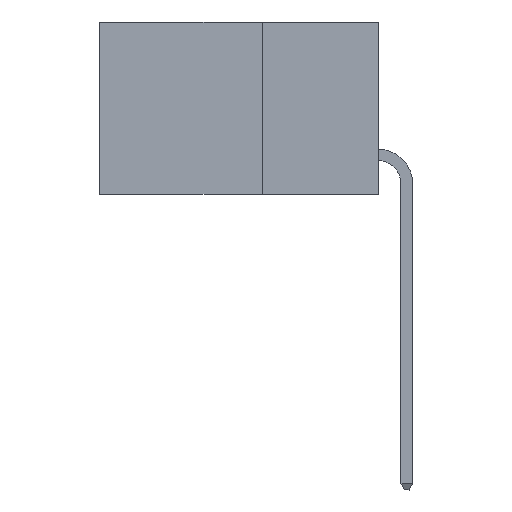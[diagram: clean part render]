
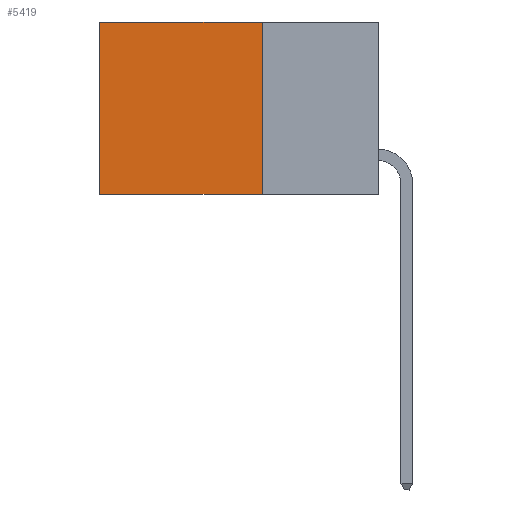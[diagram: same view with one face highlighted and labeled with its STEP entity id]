
A CAD part, left-side view. The second image highlights one B-rep face of the part: STEP entity #5419.
In plain terms, the highlighted planar face has unit normal (-1, 0, 0).
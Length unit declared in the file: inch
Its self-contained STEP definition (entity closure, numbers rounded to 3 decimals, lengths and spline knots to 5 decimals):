
#179 = VERTEX_POINT ( 'NONE', #9952 ) ;
#425 = DIRECTION ( 'NONE',  ( 0., 0., -1. ) ) ;
#601 = CARTESIAN_POINT ( 'NONE',  ( 0.298, 0.25, 0. ) ) ;
#1178 = VERTEX_POINT ( 'NONE', #8775 ) ;
#1567 = ORIENTED_EDGE ( 'NONE', *, *, #10759, .F. ) ;
#2177 = CARTESIAN_POINT ( 'NONE',  ( 0.298, 0.25, -0.37 ) ) ;
#2369 = VECTOR ( 'NONE', #10556, 39.37008 ) ;
#2895 = VERTEX_POINT ( 'NONE', #9377 ) ;
#3828 = CARTESIAN_POINT ( 'NONE',  ( 0.298, 0.25, 0. ) ) ;
#3867 = CARTESIAN_POINT ( 'NONE',  ( 0.298, 0.25, 0. ) ) ;
#4119 = FACE_OUTER_BOUND ( 'NONE', #5281, .T. ) ;
#4144 = LINE ( 'NONE', #7841, #4399 ) ;
#4399 = VECTOR ( 'NONE', #5267, 39.37008 ) ;
#4731 = EDGE_CURVE ( 'NONE', #2895, #179, #9068, .T. ) ;
#5267 = DIRECTION ( 'NONE',  ( 0., 0., -1. ) ) ;
#5281 = EDGE_LOOP ( 'NONE', ( #5848, #8081, #1567, #8512 ) ) ;
#5419 = ADVANCED_FACE ( 'NONE', ( #4119 ), #8121, .F. ) ;
#5451 = EDGE_CURVE ( 'NONE', #8329, #1178, #8147, .T. ) ;
#5575 = DIRECTION ( 'NONE',  ( 1., 0., 0. ) ) ;
#5615 = CARTESIAN_POINT ( 'NONE',  ( 0.298, 0.25, 0. ) ) ;
#5848 = ORIENTED_EDGE ( 'NONE', *, *, #10595, .T. ) ;
#5881 = VECTOR ( 'NONE', #7348, 39.37008 ) ;
#6320 = LINE ( 'NONE', #3828, #8555 ) ;
#7348 = DIRECTION ( 'NONE',  ( 0., 1., 0. ) ) ;
#7841 = CARTESIAN_POINT ( 'NONE',  ( 0.298, 0.6, 0. ) ) ;
#8081 = ORIENTED_EDGE ( 'NONE', *, *, #4731, .F. ) ;
#8121 = PLANE ( 'NONE',  #9836 ) ;
#8147 = LINE ( 'NONE', #5615, #5881 ) ;
#8329 = VERTEX_POINT ( 'NONE', #601 ) ;
#8512 = ORIENTED_EDGE ( 'NONE', *, *, #5451, .T. ) ;
#8555 = VECTOR ( 'NONE', #10592, 39.37008 ) ;
#8775 = CARTESIAN_POINT ( 'NONE',  ( 0.298, 0.6, 0. ) ) ;
#9068 = LINE ( 'NONE', #2177, #2369 ) ;
#9377 = CARTESIAN_POINT ( 'NONE',  ( 0.298, 0.25, -0.37 ) ) ;
#9836 = AXIS2_PLACEMENT_3D ( 'NONE', #3867, #5575, #425 ) ;
#9952 = CARTESIAN_POINT ( 'NONE',  ( 0.298, 0.6, -0.37 ) ) ;
#10556 = DIRECTION ( 'NONE',  ( 0., 1., 0. ) ) ;
#10592 = DIRECTION ( 'NONE',  ( 0., 0., -1. ) ) ;
#10595 = EDGE_CURVE ( 'NONE', #1178, #179, #4144, .T. ) ;
#10759 = EDGE_CURVE ( 'NONE', #8329, #2895, #6320, .T. ) ;
